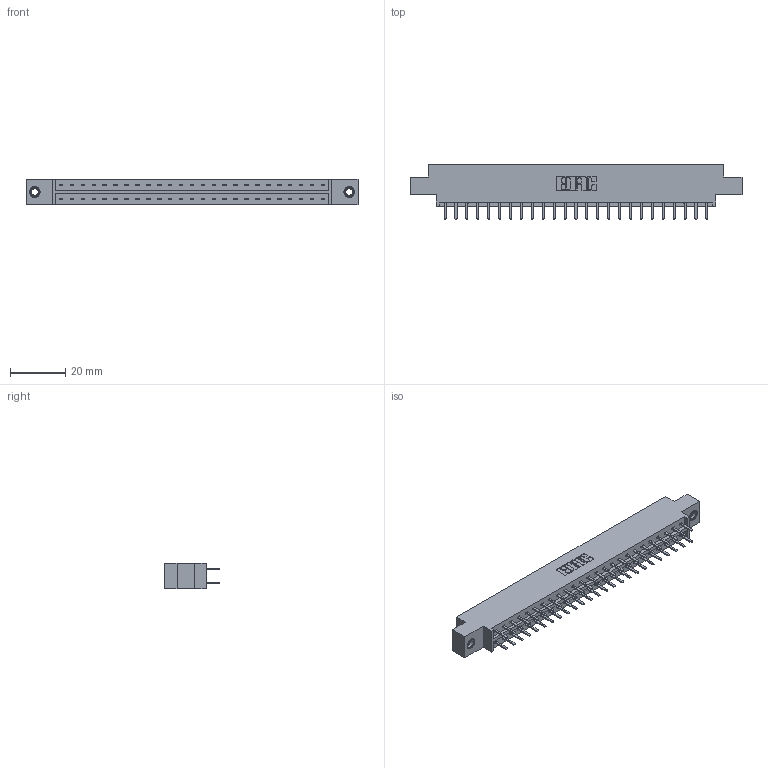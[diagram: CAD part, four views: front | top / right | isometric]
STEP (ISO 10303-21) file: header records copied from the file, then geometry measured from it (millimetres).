
FILE_DESCRIPTION (( 'STEP AP203' ), '1' );
FILE_NAME ('833-050-520-807.STEP', '2020-06-04T17:05:20', ( '' ), ( '' ), 'SwSTEP 2.0', 'SolidWorks 2020', '' );
FILE_SCHEMA (( 'CONFIG_CONTROL_DESIGN' ));
Length unit declared in the file: inch
Products named in the file (4): 345-292-001_345-293-120; 345-250-001_345-250-005-103; 833-050-520-807; 833 Part_Offset - .156 Dia - TI
Assembly tree (53 placements, depth 2):
  833-050-520-807
    833 Part_Offset - .156 Dia - TI
    345-292-001_345-293-120  x50
    345-250-001_345-250-005-103  x2
Bounding box: 120.6 x 20.02 x 9.4 mm (x, y, z)
Volume: 11890.2 mm3; surface area: 14071.3 mm2
Topology: 53 solids, 53 shells, 2978 faces, 8609 edges, 5598 vertices
Faces by surface type: plane 2006, cylinder 956, cone 12, torus 4
Entity records: 19714 total; most frequent: CARTESIAN_POINT 3285, ORIENTED_EDGE 3202, DIRECTION 2855, EDGE_CURVE 1601, LINE 1449, VECTOR 1449, VERTEX_POINT 1060, AXIS2_PLACEMENT_3D 703
